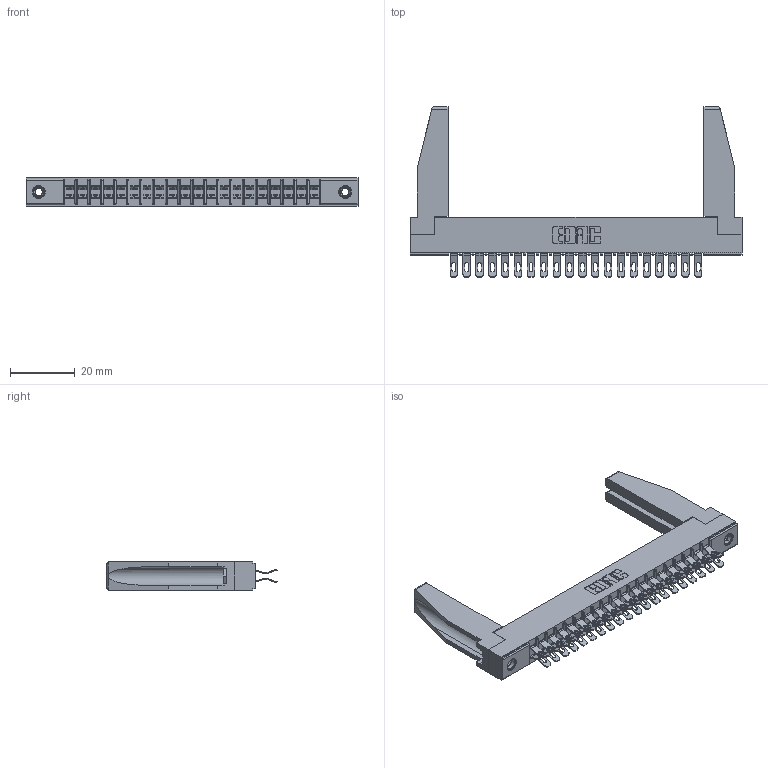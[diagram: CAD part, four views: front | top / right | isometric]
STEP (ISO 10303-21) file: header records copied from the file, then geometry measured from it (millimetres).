
FILE_DESCRIPTION (( 'STEP AP203' ), '1' );
FILE_NAME ('315-040-555-278.STEP', '2019-09-10T17:23:57', ( '' ), ( '' ), 'SwSTEP 2.0', 'SolidWorks 2016', '' );
FILE_SCHEMA (( 'CONFIG_CONTROL_DESIGN' ));
Length unit declared in the file: inch
Products named in the file (5): 307-220-078; 305 Part_.156 Dia; 315-040-555-278; 305-290-001_555; 345-250-001_345-250-001-102
Assembly tree (45 placements, depth 2):
  315-040-555-278
    305 Part_.156 Dia
    305-290-001_555  x40
    345-250-001_345-250-001-102  x2
    307-220-078  x2
Bounding box: 102.26 x 52.45 x 8.71 mm (x, y, z)
Volume: 10531.9 mm3; surface area: 16721.1 mm2
Topology: 45 solids, 45 shells, 2886 faces, 8546 edges, 5580 vertices
Faces by surface type: plane 1432, cylinder 1358, sphere 80, cone 12, torus 4
Entity records: 27396 total; most frequent: CARTESIAN_POINT 4558, ORIENTED_EDGE 4470, DIRECTION 4379, EDGE_CURVE 2235, VECTOR 1761, LINE 1761, VERTEX_POINT 1430, AXIS2_PLACEMENT_3D 1309
